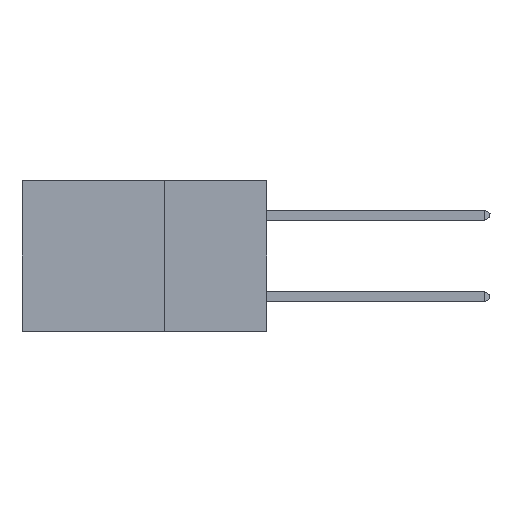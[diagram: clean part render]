
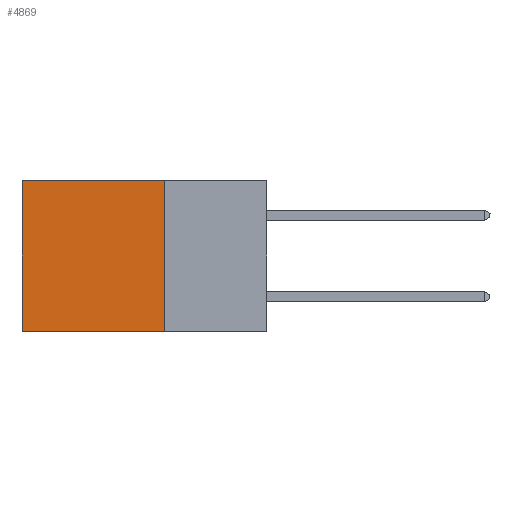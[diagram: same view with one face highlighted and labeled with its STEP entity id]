
A CAD part, left-side view. The second image highlights one B-rep face of the part: STEP entity #4869.
In plain terms, the highlighted planar face has unit normal (-1, 0, 0).
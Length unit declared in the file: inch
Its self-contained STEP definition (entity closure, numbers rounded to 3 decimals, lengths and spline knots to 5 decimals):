
#82 = ORIENTED_EDGE ( 'NONE', *, *, #8768, .F. ) ;
#114 = CARTESIAN_POINT ( 'NONE',  ( 0.2875, 0.25, 0. ) ) ;
#1023 = DIRECTION ( 'NONE',  ( 0., 1., 0. ) ) ;
#1156 = EDGE_CURVE ( 'NONE', #14640, #19274, #4235, .T. ) ;
#1252 = DIRECTION ( 'NONE',  ( 0., 0., -1. ) ) ;
#1418 = ORIENTED_EDGE ( 'NONE', *, *, #1156, .F. ) ;
#1527 = EDGE_CURVE ( 'NONE', #6827, #19274, #18492, .T. ) ;
#2640 = LINE ( 'NONE', #9140, #14472 ) ;
#2842 = VECTOR ( 'NONE', #13612, 39.37008 ) ;
#2950 = CARTESIAN_POINT ( 'NONE',  ( 0.2875, 0.25, 0. ) ) ;
#3660 = LINE ( 'NONE', #114, #9917 ) ;
#4119 = PLANE ( 'NONE',  #10966 ) ;
#4235 = LINE ( 'NONE', #20634, #18879 ) ;
#4613 = ORIENTED_EDGE ( 'NONE', *, *, #6755, .T. ) ;
#4869 = ADVANCED_FACE ( 'NONE', ( #15623 ), #4119, .F. ) ;
#6135 = DIRECTION ( 'NONE',  ( 0., 1., 0. ) ) ;
#6755 = EDGE_CURVE ( 'NONE', #10234, #6827, #2640, .T. ) ;
#6827 = VERTEX_POINT ( 'NONE', #16133 ) ;
#7626 = DIRECTION ( 'NONE',  ( 1., 0., 0. ) ) ;
#8581 = CARTESIAN_POINT ( 'NONE',  ( 0.2875, 0.25, -0.37 ) ) ;
#8768 = EDGE_CURVE ( 'NONE', #10234, #14640, #3660, .T. ) ;
#9140 = CARTESIAN_POINT ( 'NONE',  ( 0.2875, 0.25, 0. ) ) ;
#9917 = VECTOR ( 'NONE', #10175, 39.37008 ) ;
#10175 = DIRECTION ( 'NONE',  ( 0., 0., -1. ) ) ;
#10234 = VERTEX_POINT ( 'NONE', #10592 ) ;
#10592 = CARTESIAN_POINT ( 'NONE',  ( 0.2875, 0.25, 0. ) ) ;
#10966 = AXIS2_PLACEMENT_3D ( 'NONE', #2950, #7626, #1252 ) ;
#13612 = DIRECTION ( 'NONE',  ( 0., 0., -1. ) ) ;
#14472 = VECTOR ( 'NONE', #1023, 39.37008 ) ;
#14640 = VERTEX_POINT ( 'NONE', #8581 ) ;
#15212 = CARTESIAN_POINT ( 'NONE',  ( 0.2875, 0.6, -0.37 ) ) ;
#15623 = FACE_OUTER_BOUND ( 'NONE', #17899, .T. ) ;
#16133 = CARTESIAN_POINT ( 'NONE',  ( 0.2875, 0.6, 0. ) ) ;
#16475 = CARTESIAN_POINT ( 'NONE',  ( 0.2875, 0.6, 0. ) ) ;
#17173 = ORIENTED_EDGE ( 'NONE', *, *, #1527, .T. ) ;
#17899 = EDGE_LOOP ( 'NONE', ( #17173, #1418, #82, #4613 ) ) ;
#18492 = LINE ( 'NONE', #16475, #2842 ) ;
#18879 = VECTOR ( 'NONE', #6135, 39.37008 ) ;
#19274 = VERTEX_POINT ( 'NONE', #15212 ) ;
#20634 = CARTESIAN_POINT ( 'NONE',  ( 0.2875, 0.25, -0.37 ) ) ;
